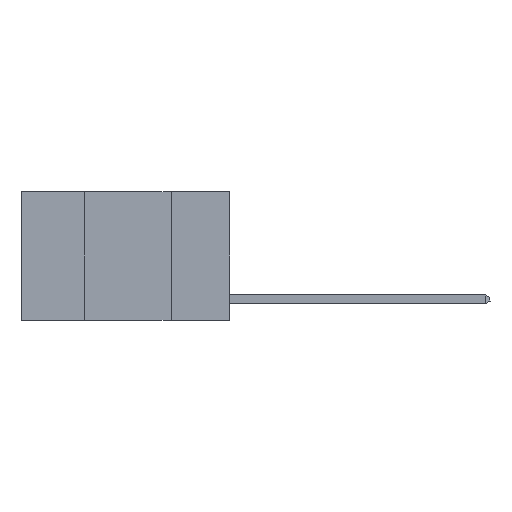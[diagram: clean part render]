
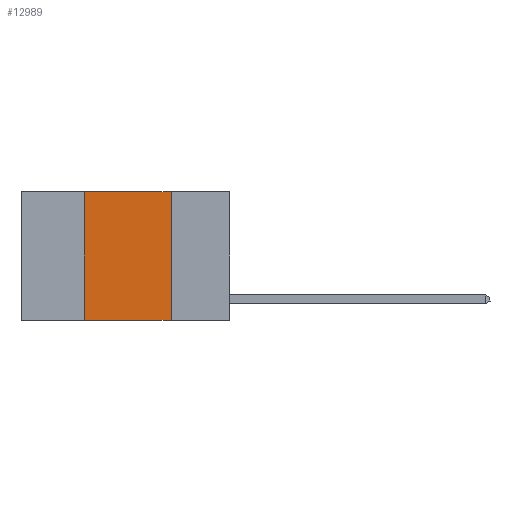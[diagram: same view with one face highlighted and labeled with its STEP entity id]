
A CAD part, left-side view. The second image highlights one B-rep face of the part: STEP entity #12989.
In plain terms, the highlighted planar face has unit normal (-1, 0, 0).
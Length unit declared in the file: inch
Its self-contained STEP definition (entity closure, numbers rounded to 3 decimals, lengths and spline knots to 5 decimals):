
#477 = DIRECTION ( 'NONE',  ( 0., -1., 0. ) ) ;
#585 = LINE ( 'NONE', #2585, #8873 ) ;
#1680 = ORIENTED_EDGE ( 'NONE', *, *, #18530, .F. ) ;
#2105 = VECTOR ( 'NONE', #11423, 39.37008 ) ;
#2293 = CARTESIAN_POINT ( 'NONE',  ( 0., 0.42, 0. ) ) ;
#2585 = CARTESIAN_POINT ( 'NONE',  ( 0., 0.6, -0.37 ) ) ;
#2839 = ORIENTED_EDGE ( 'NONE', *, *, #15381, .F. ) ;
#4420 = EDGE_CURVE ( 'NONE', #5532, #9532, #16913, .T. ) ;
#4642 = AXIS2_PLACEMENT_3D ( 'NONE', #15724, #6833, #17206 ) ;
#4984 = EDGE_LOOP ( 'NONE', ( #1680, #2839, #18769, #17654 ) ) ;
#5324 = VECTOR ( 'NONE', #477, 39.37008 ) ;
#5532 = VERTEX_POINT ( 'NONE', #6794 ) ;
#5576 = LINE ( 'NONE', #11336, #16923 ) ;
#6794 = CARTESIAN_POINT ( 'NONE',  ( 0., 0.42, -0.37 ) ) ;
#6833 = DIRECTION ( 'NONE',  ( 1., 0., 0. ) ) ;
#7896 = EDGE_CURVE ( 'NONE', #5532, #17678, #585, .T. ) ;
#8275 = PLANE ( 'NONE',  #4642 ) ;
#8873 = VECTOR ( 'NONE', #11418, 39.37008 ) ;
#9221 = LINE ( 'NONE', #18170, #5324 ) ;
#9532 = VERTEX_POINT ( 'NONE', #2293 ) ;
#9944 = CARTESIAN_POINT ( 'NONE',  ( 0., 0.42, 0. ) ) ;
#11336 = CARTESIAN_POINT ( 'NONE',  ( 0., 0.17, 0. ) ) ;
#11418 = DIRECTION ( 'NONE',  ( 0., -1., 0. ) ) ;
#11423 = DIRECTION ( 'NONE',  ( 0., 0., 1. ) ) ;
#12822 = DIRECTION ( 'NONE',  ( 0., 0., -1. ) ) ;
#12989 = ADVANCED_FACE ( 'NONE', ( #19078 ), #8275, .F. ) ;
#14770 = CARTESIAN_POINT ( 'NONE',  ( 0., 0.17, -0.37 ) ) ;
#15210 = VERTEX_POINT ( 'NONE', #17789 ) ;
#15381 = EDGE_CURVE ( 'NONE', #9532, #15210, #9221, .T. ) ;
#15724 = CARTESIAN_POINT ( 'NONE',  ( 0., 0.6, 0. ) ) ;
#16913 = LINE ( 'NONE', #9944, #2105 ) ;
#16923 = VECTOR ( 'NONE', #12822, 39.37008 ) ;
#17206 = DIRECTION ( 'NONE',  ( 0., 0., -1. ) ) ;
#17654 = ORIENTED_EDGE ( 'NONE', *, *, #7896, .T. ) ;
#17678 = VERTEX_POINT ( 'NONE', #14770 ) ;
#17789 = CARTESIAN_POINT ( 'NONE',  ( 0., 0.17, 0. ) ) ;
#18170 = CARTESIAN_POINT ( 'NONE',  ( 0., 0.6, 0. ) ) ;
#18530 = EDGE_CURVE ( 'NONE', #15210, #17678, #5576, .T. ) ;
#18769 = ORIENTED_EDGE ( 'NONE', *, *, #4420, .F. ) ;
#19078 = FACE_OUTER_BOUND ( 'NONE', #4984, .T. ) ;
